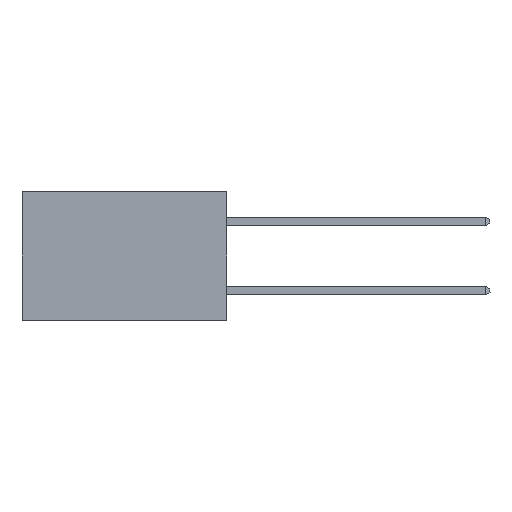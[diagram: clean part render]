
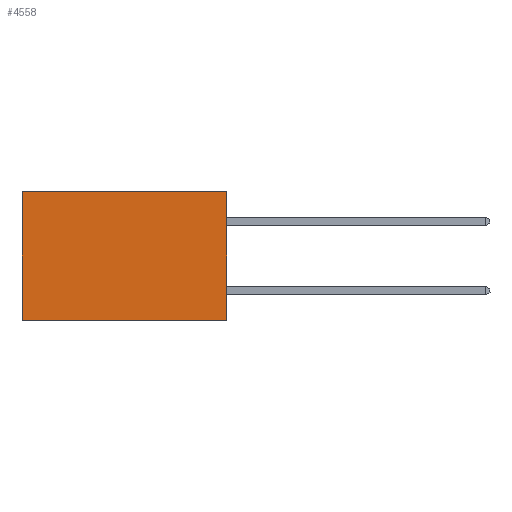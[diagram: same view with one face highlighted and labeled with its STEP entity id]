
A CAD part, left-side view. The second image highlights one B-rep face of the part: STEP entity #4558.
In plain terms, the highlighted planar face has unit normal (-1, 0, 0).
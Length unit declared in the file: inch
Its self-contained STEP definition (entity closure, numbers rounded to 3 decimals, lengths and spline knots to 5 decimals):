
#954 = VECTOR ( 'NONE', #9360, 39.37008 ) ;
#1938 = DIRECTION ( 'NONE',  ( 0., 1., 0. ) ) ;
#2586 = CARTESIAN_POINT ( 'NONE',  ( 0.277, 0., -0.37 ) ) ;
#2600 = DIRECTION ( 'NONE',  ( 0., 0., -1. ) ) ;
#2647 = CARTESIAN_POINT ( 'NONE',  ( 0.277, 0.59, -0.37 ) ) ;
#2664 = LINE ( 'NONE', #2586, #5249 ) ;
#3021 = DIRECTION ( 'NONE',  ( 0., 0., -1. ) ) ;
#3348 = ORIENTED_EDGE ( 'NONE', *, *, #6120, .T. ) ;
#3352 = ORIENTED_EDGE ( 'NONE', *, *, #9890, .T. ) ;
#3999 = AXIS2_PLACEMENT_3D ( 'NONE', #13505, #12906, #12903 ) ;
#4085 = EDGE_CURVE ( 'NONE', #6738, #12860, #9592, .T. ) ;
#4373 = EDGE_CURVE ( 'NONE', #4727, #6738, #2664, .T. ) ;
#4558 = ADVANCED_FACE ( 'NONE', ( #11364 ), #13016, .F. ) ;
#4727 = VERTEX_POINT ( 'NONE', #11727 ) ;
#5249 = VECTOR ( 'NONE', #3021, 39.37008 ) ;
#5887 = CARTESIAN_POINT ( 'NONE',  ( 0.277, 0., -0.37 ) ) ;
#6120 = EDGE_CURVE ( 'NONE', #12884, #12860, #10228, .T. ) ;
#6650 = ORIENTED_EDGE ( 'NONE', *, *, #4085, .F. ) ;
#6738 = VERTEX_POINT ( 'NONE', #5887 ) ;
#7043 = LINE ( 'NONE', #9489, #12863 ) ;
#7740 = CARTESIAN_POINT ( 'NONE',  ( 0.277, 0.59, -0.37 ) ) ;
#7781 = CARTESIAN_POINT ( 'NONE',  ( 0.277, 0.59, 0. ) ) ;
#8878 = CARTESIAN_POINT ( 'NONE',  ( 0.277, 0., -0.37 ) ) ;
#9099 = ORIENTED_EDGE ( 'NONE', *, *, #4373, .F. ) ;
#9360 = DIRECTION ( 'NONE',  ( 0., 1., 0. ) ) ;
#9489 = CARTESIAN_POINT ( 'NONE',  ( 0.277, 0., 0. ) ) ;
#9592 = LINE ( 'NONE', #8878, #954 ) ;
#9890 = EDGE_CURVE ( 'NONE', #4727, #12884, #7043, .T. ) ;
#10228 = LINE ( 'NONE', #2647, #12638 ) ;
#11364 = FACE_OUTER_BOUND ( 'NONE', #13421, .T. ) ;
#11727 = CARTESIAN_POINT ( 'NONE',  ( 0.277, 0., 0. ) ) ;
#12638 = VECTOR ( 'NONE', #2600, 39.37008 ) ;
#12860 = VERTEX_POINT ( 'NONE', #7740 ) ;
#12863 = VECTOR ( 'NONE', #1938, 39.37008 ) ;
#12884 = VERTEX_POINT ( 'NONE', #7781 ) ;
#12903 = DIRECTION ( 'NONE',  ( 0., 0., -1. ) ) ;
#12906 = DIRECTION ( 'NONE',  ( 1., 0., 0. ) ) ;
#13016 = PLANE ( 'NONE',  #3999 ) ;
#13421 = EDGE_LOOP ( 'NONE', ( #3348, #6650, #9099, #3352 ) ) ;
#13505 = CARTESIAN_POINT ( 'NONE',  ( 0.277, 0., -0.37 ) ) ;
